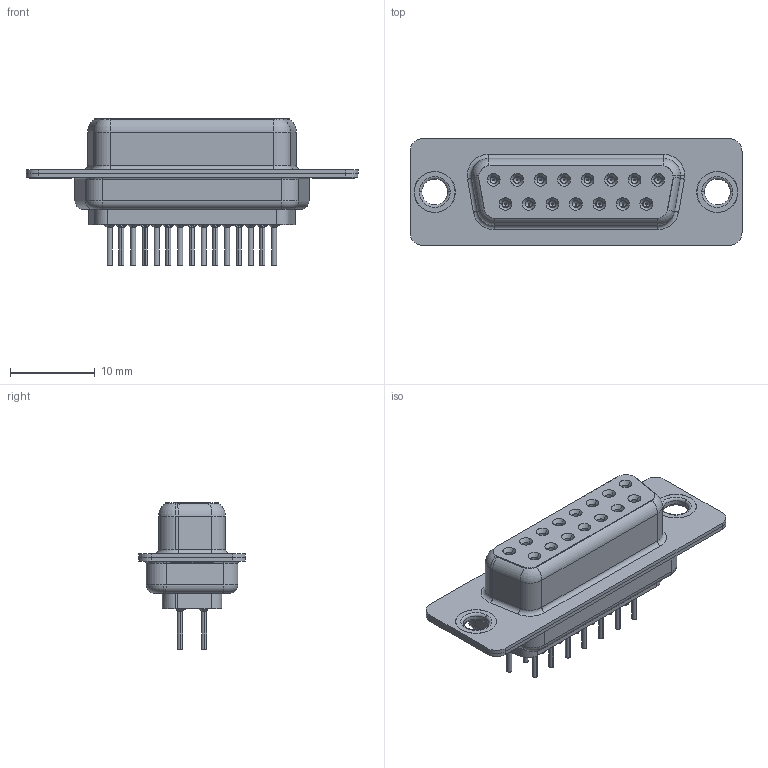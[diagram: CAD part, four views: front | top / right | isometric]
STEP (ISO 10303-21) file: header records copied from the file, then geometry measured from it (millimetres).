
FILE_DESCRIPTION (( 'STEP AP203' ), '1' );
FILE_NAME ('628-015-220-061.STEP', '2020-07-13T23:17:59', ( '' ), ( '' ), 'SwSTEP 2.0', 'SolidWorks 2020', '' );
FILE_SCHEMA (( 'CONFIG_CONTROL_DESIGN' ));
Length unit declared in the file: millimetre
Products named in the file (7): 628 Contact Row 2_20L; 628 Housing_15 LP; 628 Shell Front_15 Contacts; 628-015-220-061; 628 Contact Row 1_20L; 628 Thru Hole Rivet; 628 Shell Rear_15 Contacts
Assembly tree (20 placements, depth 2):
  628-015-220-061
    628 Housing_15 LP
    628 Shell Front_15 Contacts
    628 Shell Rear_15 Contacts
    628 Contact Row 1_20L  x8
    628 Contact Row 2_20L  x7
    628 Thru Hole Rivet  x2
Bounding box: 39.15 x 12.6 x 17.3 mm (x, y, z)
Volume: 2465.1 mm3; surface area: 6180.7 mm2
Topology: 20 solids, 20 shells, 2158 faces, 5463 edges, 3386 vertices
Faces by surface type: cylinder 616, plane 532, torus 455, bspline 300, cone 255
Entity records: 22207 total; most frequent: CARTESIAN_POINT 5775, DIRECTION 3357, ORIENTED_EDGE 3130, EDGE_CURVE 1565, AXIS2_PLACEMENT_3D 1400, VERTEX_POINT 979, CIRCLE 765, EDGE_LOOP 750
